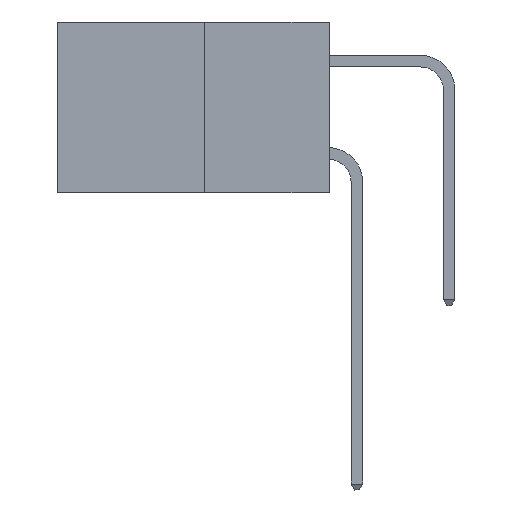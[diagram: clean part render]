
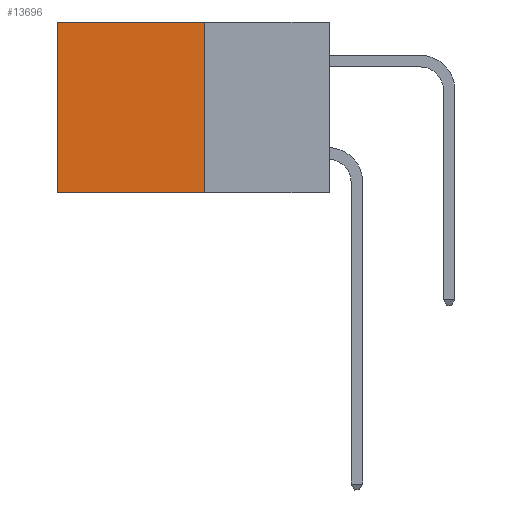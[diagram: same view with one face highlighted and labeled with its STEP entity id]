
A CAD part, left-side view. The second image highlights one B-rep face of the part: STEP entity #13696.
In plain terms, the highlighted planar face has unit normal (-1, 0, 0).
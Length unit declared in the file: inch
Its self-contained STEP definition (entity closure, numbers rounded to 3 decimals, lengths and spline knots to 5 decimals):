
#490 = EDGE_LOOP ( 'NONE', ( #4276, #5708, #1673, #14532 ) ) ;
#944 = LINE ( 'NONE', #2454, #8225 ) ;
#1002 = DIRECTION ( 'NONE',  ( 1., 0., 0. ) ) ;
#1071 = CARTESIAN_POINT ( 'NONE',  ( 0.277, 0.27, -0.37 ) ) ;
#1634 = DIRECTION ( 'NONE',  ( 0., 0., -1. ) ) ;
#1673 = ORIENTED_EDGE ( 'NONE', *, *, #13411, .F. ) ;
#1927 = FACE_OUTER_BOUND ( 'NONE', #490, .T. ) ;
#2454 = CARTESIAN_POINT ( 'NONE',  ( 0.277, 0.59, -0.37 ) ) ;
#2801 = DIRECTION ( 'NONE',  ( 0., 1., 0. ) ) ;
#3087 = CARTESIAN_POINT ( 'NONE',  ( 0.277, 0.59, 0. ) ) ;
#3998 = DIRECTION ( 'NONE',  ( 0., 0., -1. ) ) ;
#4276 = ORIENTED_EDGE ( 'NONE', *, *, #18618, .T. ) ;
#4363 = LINE ( 'NONE', #4782, #13302 ) ;
#4782 = CARTESIAN_POINT ( 'NONE',  ( 0.277, 0.27, -0.37 ) ) ;
#5562 = VERTEX_POINT ( 'NONE', #17775 ) ;
#5678 = DIRECTION ( 'NONE',  ( 0., 1., 0. ) ) ;
#5708 = ORIENTED_EDGE ( 'NONE', *, *, #13709, .F. ) ;
#7708 = CARTESIAN_POINT ( 'NONE',  ( 0.277, 0.27, -0.37 ) ) ;
#8225 = VECTOR ( 'NONE', #15132, 39.37008 ) ;
#8401 = LINE ( 'NONE', #1071, #16478 ) ;
#9013 = VERTEX_POINT ( 'NONE', #7708 ) ;
#10134 = VERTEX_POINT ( 'NONE', #12199 ) ;
#10558 = VECTOR ( 'NONE', #5678, 39.37008 ) ;
#11621 = PLANE ( 'NONE',  #18426 ) ;
#12199 = CARTESIAN_POINT ( 'NONE',  ( 0.277, 0.27, 0. ) ) ;
#13302 = VECTOR ( 'NONE', #1634, 39.37008 ) ;
#13411 = EDGE_CURVE ( 'NONE', #10134, #9013, #4363, .T. ) ;
#13696 = ADVANCED_FACE ( 'NONE', ( #1927 ), #11621, .F. ) ;
#13709 = EDGE_CURVE ( 'NONE', #9013, #5562, #8401, .T. ) ;
#14282 = VERTEX_POINT ( 'NONE', #3087 ) ;
#14315 = CARTESIAN_POINT ( 'NONE',  ( 0.277, 0.27, -0.37 ) ) ;
#14532 = ORIENTED_EDGE ( 'NONE', *, *, #17423, .T. ) ;
#15132 = DIRECTION ( 'NONE',  ( 0., 0., -1. ) ) ;
#15327 = CARTESIAN_POINT ( 'NONE',  ( 0.277, 0.27, 0. ) ) ;
#15362 = LINE ( 'NONE', #15327, #10558 ) ;
#16478 = VECTOR ( 'NONE', #2801, 39.37008 ) ;
#17423 = EDGE_CURVE ( 'NONE', #10134, #14282, #15362, .T. ) ;
#17775 = CARTESIAN_POINT ( 'NONE',  ( 0.277, 0.59, -0.37 ) ) ;
#18426 = AXIS2_PLACEMENT_3D ( 'NONE', #14315, #1002, #3998 ) ;
#18618 = EDGE_CURVE ( 'NONE', #14282, #5562, #944, .T. ) ;
